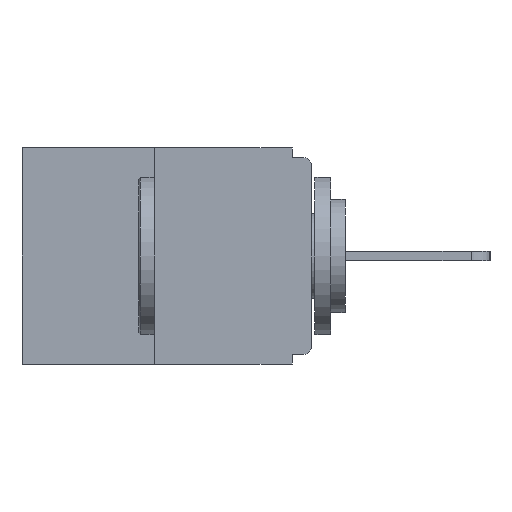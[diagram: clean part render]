
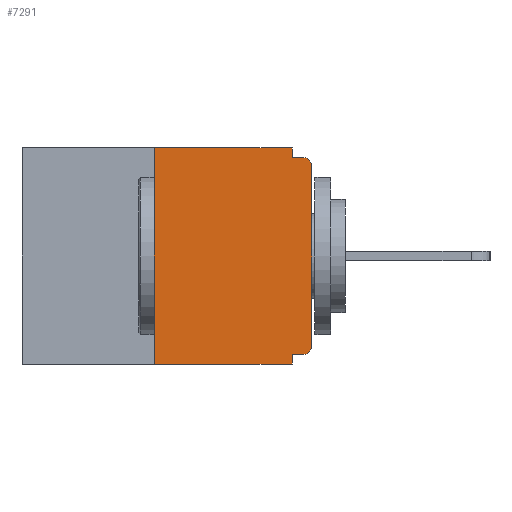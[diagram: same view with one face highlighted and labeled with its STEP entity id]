
A CAD part, left-side view. The second image highlights one B-rep face of the part: STEP entity #7291.
In plain terms, the highlighted planar face has unit normal (-1, 0, 0).
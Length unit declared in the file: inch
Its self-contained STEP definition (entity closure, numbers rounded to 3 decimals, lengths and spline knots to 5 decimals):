
#95 = CARTESIAN_POINT ( 'NONE',  ( 0., 0.031, -0.343 ) ) ;
#682 = VERTEX_POINT ( 'NONE', #5251 ) ;
#713 = CARTESIAN_POINT ( 'NONE',  ( 0., 0.25, 0. ) ) ;
#716 = DIRECTION ( 'NONE',  ( 0., 0., -1. ) ) ;
#822 = ORIENTED_EDGE ( 'NONE', *, *, #1806, .F. ) ;
#1125 = EDGE_CURVE ( 'NONE', #9212, #9084, #6839, .T. ) ;
#1142 = DIRECTION ( 'NONE',  ( 0., -1., 0. ) ) ;
#1148 = ORIENTED_EDGE ( 'NONE', *, *, #10258, .T. ) ;
#1372 = ORIENTED_EDGE ( 'NONE', *, *, #7529, .F. ) ;
#1393 = CARTESIAN_POINT ( 'NONE',  ( 0., 0., -0.03 ) ) ;
#1428 = CARTESIAN_POINT ( 'NONE',  ( 0., 0., -0.328 ) ) ;
#1573 = VERTEX_POINT ( 'NONE', #11544 ) ;
#1604 = EDGE_CURVE ( 'NONE', #9084, #11977, #5986, .T. ) ;
#1714 = VECTOR ( 'NONE', #5972, 39.37008 ) ;
#1806 = EDGE_CURVE ( 'NONE', #4912, #682, #4655, .T. ) ;
#2059 = VERTEX_POINT ( 'NONE', #11746 ) ;
#2112 = CARTESIAN_POINT ( 'NONE',  ( 0., 0.015, -0.313 ) ) ;
#2121 = VECTOR ( 'NONE', #8125, 39.37008 ) ;
#2522 = CIRCLE ( 'NONE', #9416, 0.015 ) ;
#2686 = DIRECTION ( 'NONE',  ( 0., 0., 1. ) ) ;
#2809 = VECTOR ( 'NONE', #1142, 39.37008 ) ;
#3101 = VECTOR ( 'NONE', #9049, 39.37008 ) ;
#3138 = DIRECTION ( 'NONE',  ( 0., 0., -1. ) ) ;
#3145 = VECTOR ( 'NONE', #3138, 39.37008 ) ;
#3274 = CARTESIAN_POINT ( 'NONE',  ( 0., 0.46, -0.343 ) ) ;
#3371 = ORIENTED_EDGE ( 'NONE', *, *, #13827, .F. ) ;
#4601 = LINE ( 'NONE', #13514, #1714 ) ;
#4655 = LINE ( 'NONE', #1428, #2121 ) ;
#4912 = VERTEX_POINT ( 'NONE', #13140 ) ;
#5251 = CARTESIAN_POINT ( 'NONE',  ( 0., 0.031, -0.328 ) ) ;
#5760 = CARTESIAN_POINT ( 'NONE',  ( 0., 0.46, 0. ) ) ;
#5972 = DIRECTION ( 'NONE',  ( 0., 0., 1. ) ) ;
#5986 = LINE ( 'NONE', #6281, #3145 ) ;
#6040 = ORIENTED_EDGE ( 'NONE', *, *, #13194, .F. ) ;
#6159 = VERTEX_POINT ( 'NONE', #95 ) ;
#6178 = DIRECTION ( 'NONE',  ( 0., 0., -1. ) ) ;
#6193 = AXIS2_PLACEMENT_3D ( 'NONE', #10395, #13671, #716 ) ;
#6281 = CARTESIAN_POINT ( 'NONE',  ( 0., 0.031, 0. ) ) ;
#6304 = LINE ( 'NONE', #9096, #12856 ) ;
#6674 = LINE ( 'NONE', #3274, #2809 ) ;
#6839 = LINE ( 'NONE', #11894, #7340 ) ;
#6877 = DIRECTION ( 'NONE',  ( 0., 0., -1. ) ) ;
#6899 = ORIENTED_EDGE ( 'NONE', *, *, #1125, .F. ) ;
#6979 = PLANE ( 'NONE',  #10343 ) ;
#7153 = LINE ( 'NONE', #11598, #13882 ) ;
#7188 = VERTEX_POINT ( 'NONE', #1393 ) ;
#7291 = ADVANCED_FACE ( 'NONE', ( #8276 ), #6979, .F. ) ;
#7340 = VECTOR ( 'NONE', #8634, 39.37008 ) ;
#7529 = EDGE_CURVE ( 'NONE', #11977, #1573, #10322, .T. ) ;
#7871 = EDGE_CURVE ( 'NONE', #7188, #1573, #11313, .T. ) ;
#7912 = DIRECTION ( 'NONE',  ( 1., 0., 0. ) ) ;
#8125 = DIRECTION ( 'NONE',  ( 0., 1., 0. ) ) ;
#8276 = FACE_OUTER_BOUND ( 'NONE', #11453, .T. ) ;
#8630 = CARTESIAN_POINT ( 'NONE',  ( 0., 0., -0.313 ) ) ;
#8634 = DIRECTION ( 'NONE',  ( 0., -1., 0. ) ) ;
#9049 = DIRECTION ( 'NONE',  ( 0., -1., 0. ) ) ;
#9084 = VERTEX_POINT ( 'NONE', #9262 ) ;
#9096 = CARTESIAN_POINT ( 'NONE',  ( 0., 0.25, 0. ) ) ;
#9176 = ORIENTED_EDGE ( 'NONE', *, *, #12663, .T. ) ;
#9212 = VERTEX_POINT ( 'NONE', #713 ) ;
#9262 = CARTESIAN_POINT ( 'NONE',  ( 0., 0.031, 0. ) ) ;
#9286 = ORIENTED_EDGE ( 'NONE', *, *, #11419, .T. ) ;
#9416 = AXIS2_PLACEMENT_3D ( 'NONE', #2112, #9644, #6178 ) ;
#9644 = DIRECTION ( 'NONE',  ( -1., 0., 0. ) ) ;
#10258 = EDGE_CURVE ( 'NONE', #12767, #7188, #4601, .T. ) ;
#10322 = LINE ( 'NONE', #13503, #3101 ) ;
#10343 = AXIS2_PLACEMENT_3D ( 'NONE', #5760, #7912, #6877 ) ;
#10395 = CARTESIAN_POINT ( 'NONE',  ( 0., 0.015, -0.03 ) ) ;
#10483 = DIRECTION ( 'NONE',  ( 0., 0., -1. ) ) ;
#11232 = ORIENTED_EDGE ( 'NONE', *, *, #1604, .F. ) ;
#11313 = CIRCLE ( 'NONE', #6193, 0.015 ) ;
#11419 = EDGE_CURVE ( 'NONE', #4912, #12767, #2522, .T. ) ;
#11453 = EDGE_LOOP ( 'NONE', ( #6899, #3371, #9176, #6040, #822, #9286, #1148, #12632, #1372, #11232 ) ) ;
#11544 = CARTESIAN_POINT ( 'NONE',  ( 0., 0.015, -0.015 ) ) ;
#11598 = CARTESIAN_POINT ( 'NONE',  ( 0., 0.031, -0.343 ) ) ;
#11629 = CARTESIAN_POINT ( 'NONE',  ( 0., 0.031, -0.015 ) ) ;
#11746 = CARTESIAN_POINT ( 'NONE',  ( 0., 0.25, -0.343 ) ) ;
#11894 = CARTESIAN_POINT ( 'NONE',  ( 0., 0.46, 0. ) ) ;
#11977 = VERTEX_POINT ( 'NONE', #11629 ) ;
#12632 = ORIENTED_EDGE ( 'NONE', *, *, #7871, .T. ) ;
#12663 = EDGE_CURVE ( 'NONE', #2059, #6159, #6674, .T. ) ;
#12767 = VERTEX_POINT ( 'NONE', #8630 ) ;
#12856 = VECTOR ( 'NONE', #2686, 39.37008 ) ;
#13140 = CARTESIAN_POINT ( 'NONE',  ( 0., 0.015, -0.328 ) ) ;
#13194 = EDGE_CURVE ( 'NONE', #682, #6159, #7153, .T. ) ;
#13503 = CARTESIAN_POINT ( 'NONE',  ( 0., 0., -0.015 ) ) ;
#13514 = CARTESIAN_POINT ( 'NONE',  ( 0., 0., 0. ) ) ;
#13671 = DIRECTION ( 'NONE',  ( -1., 0., 0. ) ) ;
#13827 = EDGE_CURVE ( 'NONE', #2059, #9212, #6304, .T. ) ;
#13882 = VECTOR ( 'NONE', #10483, 39.37008 ) ;
